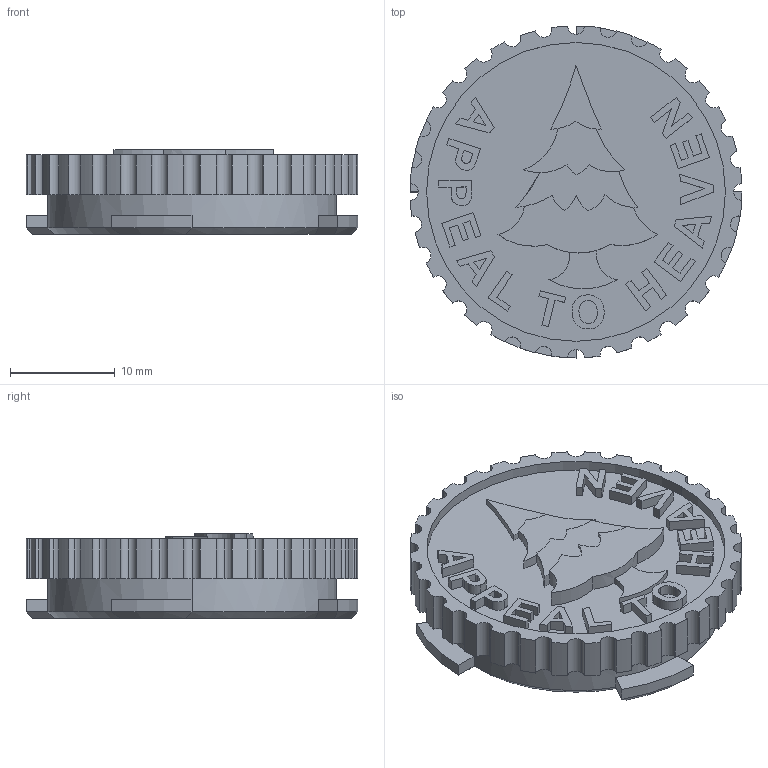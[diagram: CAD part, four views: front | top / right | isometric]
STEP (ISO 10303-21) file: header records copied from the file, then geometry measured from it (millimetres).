
FILE_DESCRIPTION (( 'STEP AP203' ), '1' );
FILE_NAME ('AF-HF-TK-PRT-006-STEP_APPEAL_TO_HEAVEN.STEP', '2020-12-04T14:33:59', ( '' ), ( '' ), 'SwSTEP 2.0', 'SolidWorks 2018', '' );
FILE_SCHEMA (( 'CONFIG_CONTROL_DESIGN' ));
Length unit declared in the file: inch
Products named in the file (1): AF-HF-TK-PRT-006-STEP_APPEAL_TO_HEAVEN
Bounding box: 31.75 x 31.75 x 8.12 mm (x, y, z)
Volume: 3870.3 mm3; surface area: 2929.7 mm2
Topology: 1 solids, 1 shells, 338 faces, 906 edges, 594 vertices
Faces by surface type: plane 177, cylinder 122, bspline 24, cone 13, sphere 2
Entity records: 11852 total; most frequent: CARTESIAN_POINT 3255, ORIENTED_EDGE 1812, DIRECTION 1739, EDGE_CURVE 906, VERTEX_POINT 594, AXIS2_PLACEMENT_3D 582, VECTOR 575, LINE 575
